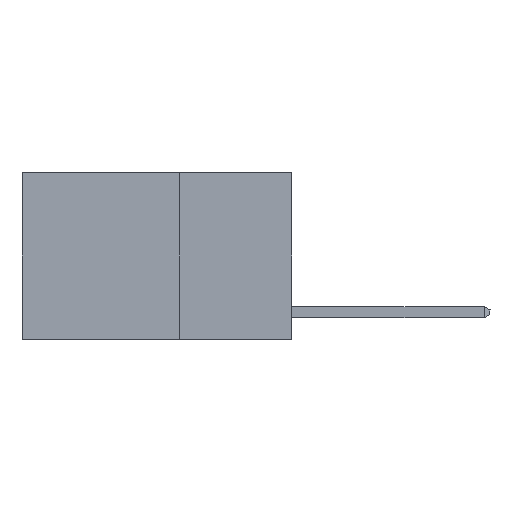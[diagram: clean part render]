
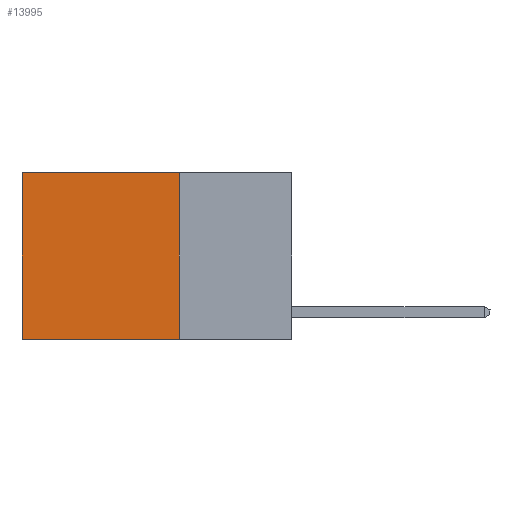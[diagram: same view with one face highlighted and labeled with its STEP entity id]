
A CAD part, left-side view. The second image highlights one B-rep face of the part: STEP entity #13995.
In plain terms, the highlighted planar face has unit normal (-1, 0, 0).
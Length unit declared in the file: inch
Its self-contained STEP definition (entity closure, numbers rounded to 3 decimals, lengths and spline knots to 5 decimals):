
#186 = EDGE_LOOP ( 'NONE', ( #15852, #13575, #7812, #5735 ) ) ;
#225 = CARTESIAN_POINT ( 'NONE',  ( 0.2625, 0.25, -0.37 ) ) ;
#291 = DIRECTION ( 'NONE',  ( 0., 0., -1. ) ) ;
#759 = CARTESIAN_POINT ( 'NONE',  ( 0.2625, 0.25, 0. ) ) ;
#1436 = DIRECTION ( 'NONE',  ( 0., 1., 0. ) ) ;
#2619 = CARTESIAN_POINT ( 'NONE',  ( 0.2625, 0.25, -0.37 ) ) ;
#2950 = VERTEX_POINT ( 'NONE', #12604 ) ;
#2990 = LINE ( 'NONE', #8404, #9803 ) ;
#4429 = DIRECTION ( 'NONE',  ( 0., 1., 0. ) ) ;
#4682 = DIRECTION ( 'NONE',  ( 0., 0., -1. ) ) ;
#5735 = ORIENTED_EDGE ( 'NONE', *, *, #13807, .T. ) ;
#6903 = CARTESIAN_POINT ( 'NONE',  ( 0.2625, 0.6, -0.37 ) ) ;
#7653 = FACE_OUTER_BOUND ( 'NONE', #186, .T. ) ;
#7812 = ORIENTED_EDGE ( 'NONE', *, *, #14714, .F. ) ;
#7816 = VERTEX_POINT ( 'NONE', #12141 ) ;
#8404 = CARTESIAN_POINT ( 'NONE',  ( 0.2625, 0.6, 0. ) ) ;
#8668 = EDGE_CURVE ( 'NONE', #7816, #9746, #2990, .T. ) ;
#9344 = VECTOR ( 'NONE', #291, 39.37008 ) ;
#9746 = VERTEX_POINT ( 'NONE', #6903 ) ;
#9803 = VECTOR ( 'NONE', #13627, 39.37008 ) ;
#10407 = VECTOR ( 'NONE', #4429, 39.37008 ) ;
#10466 = LINE ( 'NONE', #225, #14830 ) ;
#10866 = CARTESIAN_POINT ( 'NONE',  ( 0.2625, 0.25, 0. ) ) ;
#11164 = PLANE ( 'NONE',  #12326 ) ;
#12141 = CARTESIAN_POINT ( 'NONE',  ( 0.2625, 0.6, 0. ) ) ;
#12326 = AXIS2_PLACEMENT_3D ( 'NONE', #759, #16371, #4682 ) ;
#12604 = CARTESIAN_POINT ( 'NONE',  ( 0.2625, 0.25, 0. ) ) ;
#13388 = CARTESIAN_POINT ( 'NONE',  ( 0.2625, 0.25, 0. ) ) ;
#13575 = ORIENTED_EDGE ( 'NONE', *, *, #15363, .F. ) ;
#13627 = DIRECTION ( 'NONE',  ( 0., 0., -1. ) ) ;
#13807 = EDGE_CURVE ( 'NONE', #2950, #7816, #16204, .T. ) ;
#13995 = ADVANCED_FACE ( 'NONE', ( #7653 ), #11164, .F. ) ;
#14714 = EDGE_CURVE ( 'NONE', #2950, #15903, #15925, .T. ) ;
#14830 = VECTOR ( 'NONE', #1436, 39.37008 ) ;
#15363 = EDGE_CURVE ( 'NONE', #15903, #9746, #10466, .T. ) ;
#15852 = ORIENTED_EDGE ( 'NONE', *, *, #8668, .T. ) ;
#15903 = VERTEX_POINT ( 'NONE', #2619 ) ;
#15925 = LINE ( 'NONE', #10866, #9344 ) ;
#16204 = LINE ( 'NONE', #13388, #10407 ) ;
#16371 = DIRECTION ( 'NONE',  ( 1., 0., 0. ) ) ;
